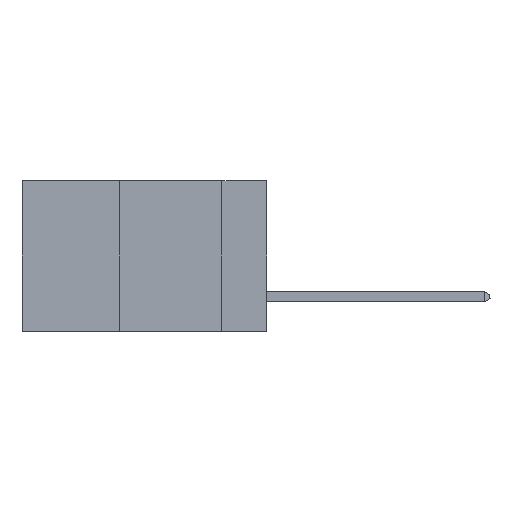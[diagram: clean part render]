
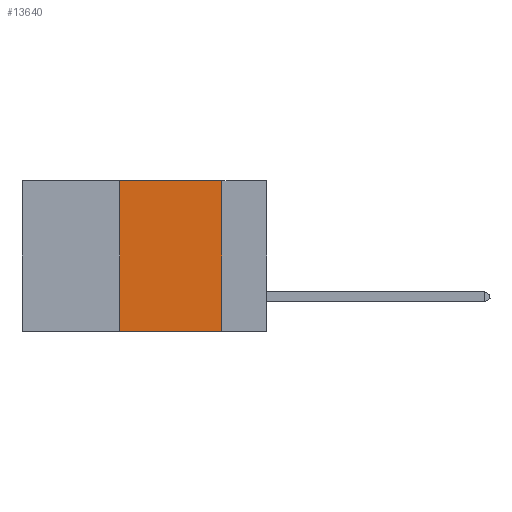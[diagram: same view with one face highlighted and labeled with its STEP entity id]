
A CAD part, left-side view. The second image highlights one B-rep face of the part: STEP entity #13640.
In plain terms, the highlighted planar face has unit normal (-1, 0, 0).
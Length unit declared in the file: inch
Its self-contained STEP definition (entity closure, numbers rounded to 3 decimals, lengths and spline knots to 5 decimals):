
#183 = VECTOR ( 'NONE', #6440, 39.37008 ) ;
#920 = EDGE_CURVE ( 'NONE', #6105, #10737, #16317, .T. ) ;
#1979 = LINE ( 'NONE', #19486, #5328 ) ;
#3407 = LINE ( 'NONE', #5331, #19537 ) ;
#3446 = CARTESIAN_POINT ( 'NONE',  ( 0., 0.11, 0. ) ) ;
#4156 = VERTEX_POINT ( 'NONE', #19247 ) ;
#5328 = VECTOR ( 'NONE', #9026, 39.37008 ) ;
#5331 = CARTESIAN_POINT ( 'NONE',  ( 0., 0.6, 0. ) ) ;
#5677 = DIRECTION ( 'NONE',  ( 0., 0., -1. ) ) ;
#6105 = VERTEX_POINT ( 'NONE', #3446 ) ;
#6127 = CARTESIAN_POINT ( 'NONE',  ( 0., 0.36, 0. ) ) ;
#6394 = CARTESIAN_POINT ( 'NONE',  ( 0., 0.11, -0.37 ) ) ;
#6440 = DIRECTION ( 'NONE',  ( 0., 0., -1. ) ) ;
#6502 = EDGE_CURVE ( 'NONE', #4156, #10737, #18692, .T. ) ;
#6731 = ORIENTED_EDGE ( 'NONE', *, *, #920, .F. ) ;
#8133 = VECTOR ( 'NONE', #22177, 39.37008 ) ;
#9026 = DIRECTION ( 'NONE',  ( 0., 0., 1. ) ) ;
#9115 = DIRECTION ( 'NONE',  ( 1., 0., 0. ) ) ;
#9135 = AXIS2_PLACEMENT_3D ( 'NONE', #12897, #9115, #5677 ) ;
#9854 = ORIENTED_EDGE ( 'NONE', *, *, #22099, .F. ) ;
#10200 = CARTESIAN_POINT ( 'NONE',  ( 0., 0.11, 0. ) ) ;
#10737 = VERTEX_POINT ( 'NONE', #6394 ) ;
#10816 = PLANE ( 'NONE',  #9135 ) ;
#11528 = ORIENTED_EDGE ( 'NONE', *, *, #6502, .T. ) ;
#12406 = EDGE_CURVE ( 'NONE', #4156, #22561, #1979, .T. ) ;
#12788 = FACE_OUTER_BOUND ( 'NONE', #16765, .T. ) ;
#12897 = CARTESIAN_POINT ( 'NONE',  ( 0., 0.6, 0. ) ) ;
#13640 = ADVANCED_FACE ( 'NONE', ( #12788 ), #10816, .F. ) ;
#14190 = DIRECTION ( 'NONE',  ( 0., -1., 0. ) ) ;
#15003 = CARTESIAN_POINT ( 'NONE',  ( 0., 0.6, -0.37 ) ) ;
#15947 = ORIENTED_EDGE ( 'NONE', *, *, #12406, .F. ) ;
#16317 = LINE ( 'NONE', #10200, #183 ) ;
#16765 = EDGE_LOOP ( 'NONE', ( #6731, #9854, #15947, #11528 ) ) ;
#18692 = LINE ( 'NONE', #15003, #8133 ) ;
#19247 = CARTESIAN_POINT ( 'NONE',  ( 0., 0.36, -0.37 ) ) ;
#19486 = CARTESIAN_POINT ( 'NONE',  ( 0., 0.36, 0. ) ) ;
#19537 = VECTOR ( 'NONE', #14190, 39.37008 ) ;
#22099 = EDGE_CURVE ( 'NONE', #22561, #6105, #3407, .T. ) ;
#22177 = DIRECTION ( 'NONE',  ( 0., -1., 0. ) ) ;
#22561 = VERTEX_POINT ( 'NONE', #6127 ) ;
